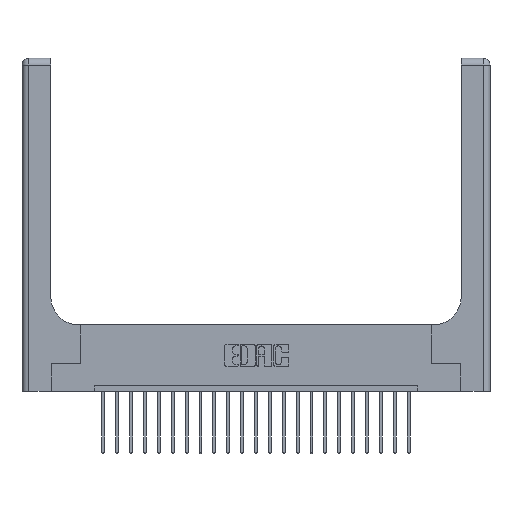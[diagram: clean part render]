
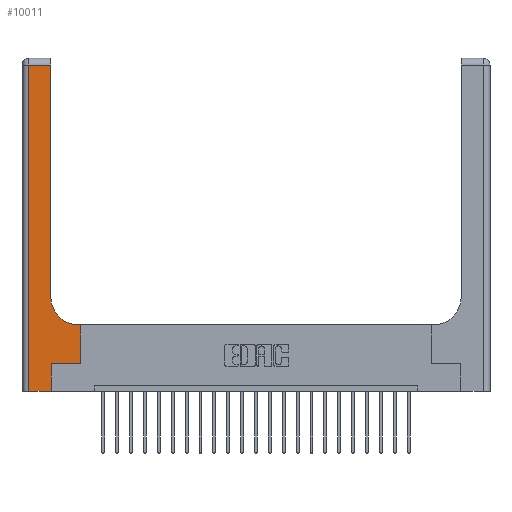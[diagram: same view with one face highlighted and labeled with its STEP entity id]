
A CAD part, top view. The second image highlights one B-rep face of the part: STEP entity #10011.
In plain terms, the highlighted planar face has unit normal (0, 0, 1).
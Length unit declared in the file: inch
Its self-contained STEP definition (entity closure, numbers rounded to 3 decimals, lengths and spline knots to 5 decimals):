
#31 = LINE ( 'NONE', #15714, #8012 ) ;
#128 = ORIENTED_EDGE ( 'NONE', *, *, #18360, .T. ) ;
#1299 = DIRECTION ( 'NONE',  ( 0., 0., -1. ) ) ;
#1310 = VECTOR ( 'NONE', #14015, 39.37008 ) ;
#1430 = CARTESIAN_POINT ( 'NONE',  ( 0.06, 2.94, 0.37 ) ) ;
#1574 = EDGE_CURVE ( 'NONE', #2635, #3852, #14884, .T. ) ;
#1716 = CARTESIAN_POINT ( 'NONE',  ( 0.51, 0.6, 0.37 ) ) ;
#1862 = ORIENTED_EDGE ( 'NONE', *, *, #1574, .T. ) ;
#2152 = ORIENTED_EDGE ( 'NONE', *, *, #17724, .T. ) ;
#2635 = VERTEX_POINT ( 'NONE', #21824 ) ;
#2953 = ORIENTED_EDGE ( 'NONE', *, *, #9258, .T. ) ;
#3631 = ORIENTED_EDGE ( 'NONE', *, *, #10990, .T. ) ;
#3649 = CARTESIAN_POINT ( 'NONE',  ( 0.26, 3., 0.37 ) ) ;
#3852 = VERTEX_POINT ( 'NONE', #1430 ) ;
#4624 = ORIENTED_EDGE ( 'NONE', *, *, #6085, .T. ) ;
#5154 = ORIENTED_EDGE ( 'NONE', *, *, #15745, .T. ) ;
#5358 = DIRECTION ( 'NONE',  ( 0., -1., 0. ) ) ;
#5478 = LINE ( 'NONE', #3649, #1310 ) ;
#5860 = DIRECTION ( 'NONE',  ( 0., 0., -1. ) ) ;
#5894 = LINE ( 'NONE', #12858, #19467 ) ;
#6006 = VERTEX_POINT ( 'NONE', #11966 ) ;
#6085 = EDGE_CURVE ( 'NONE', #6006, #2635, #5478, .T. ) ;
#6315 = CARTESIAN_POINT ( 'NONE',  ( 0.26, 0.6, 0.37 ) ) ;
#6655 = LINE ( 'NONE', #6315, #8071 ) ;
#6665 = DIRECTION ( 'NONE',  ( -1., 0., 0. ) ) ;
#6973 = VECTOR ( 'NONE', #18395, 39.37008 ) ;
#7884 = CARTESIAN_POINT ( 'NONE',  ( 0.528, 0.25, 0.37 ) ) ;
#8012 = VECTOR ( 'NONE', #5358, 39.37008 ) ;
#8071 = VECTOR ( 'NONE', #13274, 39.37008 ) ;
#8168 = CARTESIAN_POINT ( 'NONE',  ( 0.528, 0.25, 0.37 ) ) ;
#9051 = VERTEX_POINT ( 'NONE', #21274 ) ;
#9258 = EDGE_CURVE ( 'NONE', #13223, #10394, #5894, .T. ) ;
#9375 = LINE ( 'NONE', #14940, #22259 ) ;
#9490 = VERTEX_POINT ( 'NONE', #10576 ) ;
#9753 = DIRECTION ( 'NONE',  ( 1., 0., 0. ) ) ;
#9770 = VECTOR ( 'NONE', #6665, 39.37008 ) ;
#10011 = ADVANCED_FACE ( 'NONE', ( #16784 ), #18599, .F. ) ;
#10394 = VERTEX_POINT ( 'NONE', #7884 ) ;
#10576 = CARTESIAN_POINT ( 'NONE',  ( 0.06, 0., 0.37 ) ) ;
#10990 = EDGE_CURVE ( 'NONE', #15693, #6006, #14806, .T. ) ;
#11966 = CARTESIAN_POINT ( 'NONE',  ( 0.26, 0.85, 0.37 ) ) ;
#12288 = AXIS2_PLACEMENT_3D ( 'NONE', #14861, #5860, #9753 ) ;
#12858 = CARTESIAN_POINT ( 'NONE',  ( 0.265, 0.25, 0.37 ) ) ;
#12888 = DIRECTION ( 'NONE',  ( 0., 1., 0. ) ) ;
#13144 = CARTESIAN_POINT ( 'NONE',  ( 0., 0., 0.37 ) ) ;
#13223 = VERTEX_POINT ( 'NONE', #16750 ) ;
#13274 = DIRECTION ( 'NONE',  ( -1., 0., 0. ) ) ;
#13384 = LINE ( 'NONE', #8168, #6973 ) ;
#13500 = CARTESIAN_POINT ( 'NONE',  ( 0.265, 0., 0.37 ) ) ;
#13584 = DIRECTION ( 'NONE',  ( -1., 0., 0. ) ) ;
#14015 = DIRECTION ( 'NONE',  ( 0., 1., 0. ) ) ;
#14806 = CIRCLE ( 'NONE', #12288, 0.25 ) ;
#14861 = CARTESIAN_POINT ( 'NONE',  ( 0.51, 0.85, 0.37 ) ) ;
#14884 = LINE ( 'NONE', #22015, #9770 ) ;
#14940 = CARTESIAN_POINT ( 'NONE',  ( 0.265, 0., 0.37 ) ) ;
#14963 = DIRECTION ( 'NONE',  ( 1., 0., 0. ) ) ;
#15184 = CARTESIAN_POINT ( 'NONE',  ( 0., 3., 0.37 ) ) ;
#15693 = VERTEX_POINT ( 'NONE', #1716 ) ;
#15714 = CARTESIAN_POINT ( 'NONE',  ( 0.06, 3., 0.37 ) ) ;
#15745 = EDGE_CURVE ( 'NONE', #3852, #9490, #31, .T. ) ;
#15931 = EDGE_LOOP ( 'NONE', ( #4624, #1862, #5154, #128, #19516, #2953, #20501, #2152, #3631 ) ) ;
#16750 = CARTESIAN_POINT ( 'NONE',  ( 0.265, 0.25, 0.37 ) ) ;
#16784 = FACE_OUTER_BOUND ( 'NONE', #15931, .T. ) ;
#17651 = EDGE_CURVE ( 'NONE', #10394, #9051, #13384, .T. ) ;
#17724 = EDGE_CURVE ( 'NONE', #9051, #15693, #6655, .T. ) ;
#18360 = EDGE_CURVE ( 'NONE', #9490, #22195, #20187, .T. ) ;
#18395 = DIRECTION ( 'NONE',  ( 0., 1., 0. ) ) ;
#18599 = PLANE ( 'NONE',  #22394 ) ;
#18615 = VECTOR ( 'NONE', #14963, 39.37008 ) ;
#18867 = EDGE_CURVE ( 'NONE', #22195, #13223, #9375, .T. ) ;
#19467 = VECTOR ( 'NONE', #19780, 39.37008 ) ;
#19516 = ORIENTED_EDGE ( 'NONE', *, *, #18867, .T. ) ;
#19780 = DIRECTION ( 'NONE',  ( 1., 0., 0. ) ) ;
#20187 = LINE ( 'NONE', #13144, #18615 ) ;
#20501 = ORIENTED_EDGE ( 'NONE', *, *, #17651, .T. ) ;
#21274 = CARTESIAN_POINT ( 'NONE',  ( 0.528, 0.6, 0.37 ) ) ;
#21824 = CARTESIAN_POINT ( 'NONE',  ( 0.26, 2.94, 0.37 ) ) ;
#22015 = CARTESIAN_POINT ( 'NONE',  ( 0., 2.94, 0.37 ) ) ;
#22195 = VERTEX_POINT ( 'NONE', #13500 ) ;
#22259 = VECTOR ( 'NONE', #12888, 39.37008 ) ;
#22394 = AXIS2_PLACEMENT_3D ( 'NONE', #15184, #1299, #13584 ) ;
